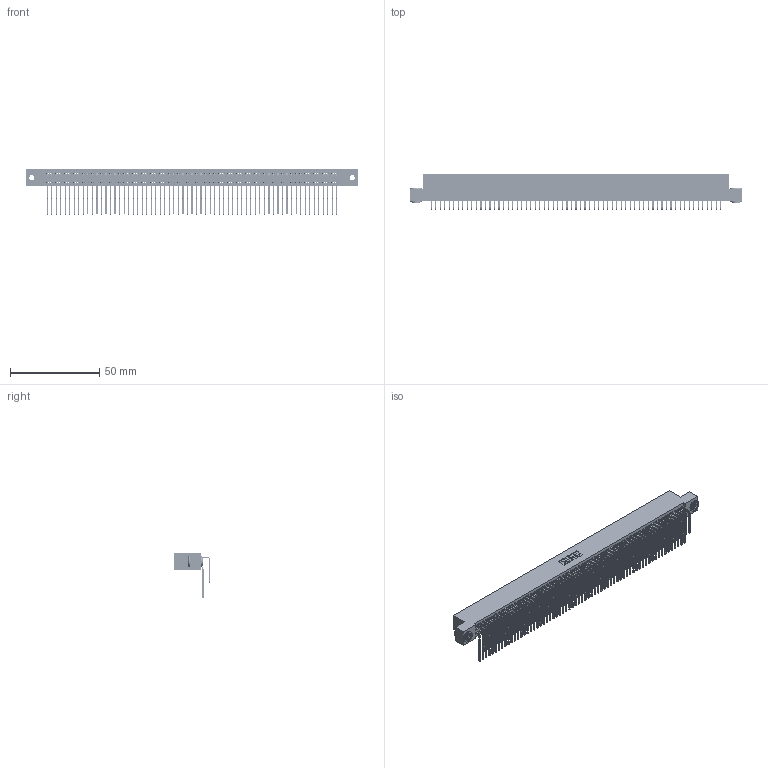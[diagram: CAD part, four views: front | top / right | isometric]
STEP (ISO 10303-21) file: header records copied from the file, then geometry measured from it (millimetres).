
FILE_DESCRIPTION (( 'STEP AP203' ), '1' );
FILE_NAME ('395-130-559-203.STEP', '2019-10-29T00:52:04', ( '' ), ( '' ), 'SwSTEP 2.0', 'SolidWorks 2016', '' );
FILE_SCHEMA (( 'CONFIG_CONTROL_DESIGN' ));
Length unit declared in the file: inch
Products named in the file (5): 345 Part_Flush Mounting Lugs - 0.156 Dia-TH; 345-292-001_558 559 Tail - 1; 345-292-001_559 Tail - 2; 345-250-002_345-250-002-102; 395-130-559-203
Assembly tree (133 placements, depth 2):
  395-130-559-203
    345 Part_Flush Mounting Lugs - 0.156 Dia-TH
    345-292-001_558 559 Tail - 1  x65
    345-292-001_559 Tail - 2  x65
    345-250-002_345-250-002-102  x2
Bounding box: 186.31 x 20.56 x 25.53 mm (x, y, z)
Volume: 19081.1 mm3; surface area: 32381.8 mm2
Topology: 133 solids, 133 shells, 6924 faces, 20567 edges, 13534 vertices
Faces by surface type: plane 4640, cylinder 2276, cone 8
Entity records: 50206 total; most frequent: CARTESIAN_POINT 8414, ORIENTED_EDGE 8290, DIRECTION 7395, EDGE_CURVE 4145, VECTOR 3689, LINE 3689, VERTEX_POINT 2758, AXIS2_PLACEMENT_3D 1853
